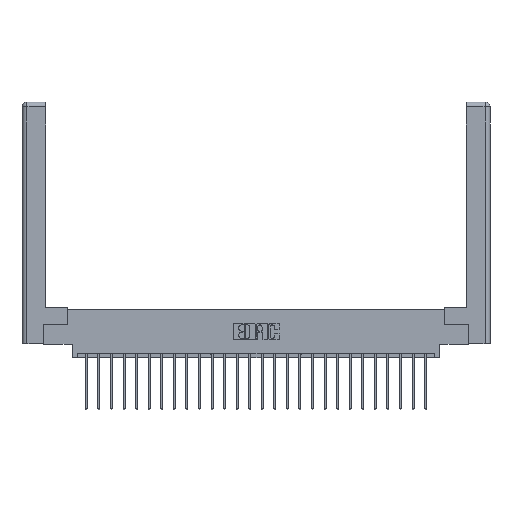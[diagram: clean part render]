
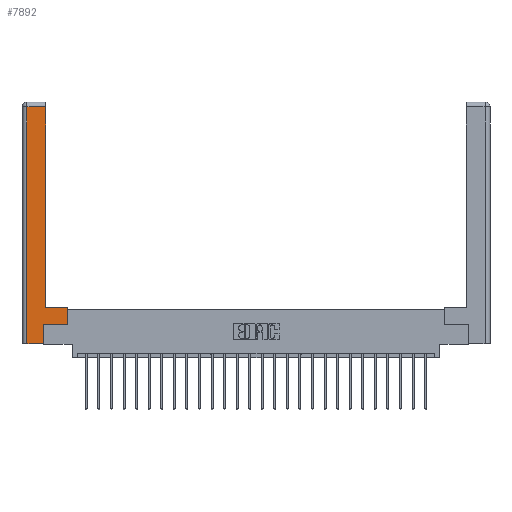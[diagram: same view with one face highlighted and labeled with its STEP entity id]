
A CAD part, top view. The second image highlights one B-rep face of the part: STEP entity #7892.
In plain terms, the highlighted planar face has unit normal (0, 0, 1).
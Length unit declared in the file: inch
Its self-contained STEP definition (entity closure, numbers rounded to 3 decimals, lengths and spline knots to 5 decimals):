
#129 = VECTOR ( 'NONE', #10155, 39.37008 ) ;
#298 = VERTEX_POINT ( 'NONE', #1023 ) ;
#377 = VECTOR ( 'NONE', #16266, 39.37008 ) ;
#504 = CARTESIAN_POINT ( 'NONE',  ( 0.295, 0.45, 0. ) ) ;
#932 = DIRECTION ( 'NONE',  ( 1., 0., 0. ) ) ;
#964 = DIRECTION ( 'NONE',  ( 1., 0., 0. ) ) ;
#1023 = CARTESIAN_POINT ( 'NONE',  ( 0.565, 0.245, 0. ) ) ;
#1202 = VECTOR ( 'NONE', #964, 39.37008 ) ;
#1464 = FACE_OUTER_BOUND ( 'NONE', #13338, .T. ) ;
#1523 = CARTESIAN_POINT ( 'NONE',  ( 0.295, 2.94, 0. ) ) ;
#1764 = VERTEX_POINT ( 'NONE', #23637 ) ;
#1987 = EDGE_CURVE ( 'NONE', #4598, #22615, #16367, .T. ) ;
#2951 = LINE ( 'NONE', #18261, #129 ) ;
#4598 = VERTEX_POINT ( 'NONE', #504 ) ;
#4826 = ORIENTED_EDGE ( 'NONE', *, *, #24903, .T. ) ;
#5138 = EDGE_CURVE ( 'NONE', #13540, #10791, #15281, .T. ) ;
#5182 = LINE ( 'NONE', #15343, #7731 ) ;
#5396 = CARTESIAN_POINT ( 'NONE',  ( 0.0615, 2.94, 0. ) ) ;
#7731 = VECTOR ( 'NONE', #932, 39.37008 ) ;
#7892 = ADVANCED_FACE ( 'NONE', ( #1464 ), #26031, .F. ) ;
#8048 = DIRECTION ( 'NONE',  ( 0., 1., 0. ) ) ;
#8548 = DIRECTION ( 'NONE',  ( 0., 0., -1. ) ) ;
#9258 = LINE ( 'NONE', #14224, #377 ) ;
#9481 = DIRECTION ( 'NONE',  ( -1., 0., 0. ) ) ;
#10155 = DIRECTION ( 'NONE',  ( 0., -1., 0. ) ) ;
#10300 = VECTOR ( 'NONE', #8048, 39.37008 ) ;
#10791 = VERTEX_POINT ( 'NONE', #21172 ) ;
#11776 = VECTOR ( 'NONE', #22174, 39.37008 ) ;
#11961 = VECTOR ( 'NONE', #25441, 39.37008 ) ;
#11969 = VERTEX_POINT ( 'NONE', #19261 ) ;
#12042 = ORIENTED_EDGE ( 'NONE', *, *, #26000, .T. ) ;
#12096 = CARTESIAN_POINT ( 'NONE',  ( 0.295, 3., 0. ) ) ;
#12548 = ORIENTED_EDGE ( 'NONE', *, *, #1987, .T. ) ;
#13338 = EDGE_LOOP ( 'NONE', ( #12548, #18066, #20250, #12042, #24598, #20598, #4826, #26020 ) ) ;
#13540 = VERTEX_POINT ( 'NONE', #19562 ) ;
#13915 = EDGE_CURVE ( 'NONE', #10791, #298, #13944, .T. ) ;
#13944 = LINE ( 'NONE', #25064, #1202 ) ;
#14224 = CARTESIAN_POINT ( 'NONE',  ( 0.295, 0.45, 0. ) ) ;
#14632 = EDGE_CURVE ( 'NONE', #22615, #1764, #26293, .T. ) ;
#14956 = CARTESIAN_POINT ( 'NONE',  ( 0.565, 0.45, 0. ) ) ;
#15281 = LINE ( 'NONE', #22257, #11776 ) ;
#15343 = CARTESIAN_POINT ( 'NONE',  ( 0.265, 0., 0. ) ) ;
#16112 = VECTOR ( 'NONE', #9481, 39.37008 ) ;
#16266 = DIRECTION ( 'NONE',  ( -1., 0., 0. ) ) ;
#16367 = LINE ( 'NONE', #12096, #10300 ) ;
#17189 = CARTESIAN_POINT ( 'NONE',  ( 0.565, 0.45, 0. ) ) ;
#18066 = ORIENTED_EDGE ( 'NONE', *, *, #14632, .T. ) ;
#18261 = CARTESIAN_POINT ( 'NONE',  ( 0.0615, 0., 0. ) ) ;
#18473 = EDGE_CURVE ( 'NONE', #1764, #11969, #2951, .T. ) ;
#19261 = CARTESIAN_POINT ( 'NONE',  ( 0.0615, 0., 0. ) ) ;
#19562 = CARTESIAN_POINT ( 'NONE',  ( 0.265, 0., 0. ) ) ;
#20184 = EDGE_CURVE ( 'NONE', #22266, #4598, #9258, .T. ) ;
#20250 = ORIENTED_EDGE ( 'NONE', *, *, #18473, .T. ) ;
#20385 = CARTESIAN_POINT ( 'NONE',  ( 0., 0., 0. ) ) ;
#20598 = ORIENTED_EDGE ( 'NONE', *, *, #13915, .T. ) ;
#20929 = DIRECTION ( 'NONE',  ( -1., 0., 0. ) ) ;
#21172 = CARTESIAN_POINT ( 'NONE',  ( 0.265, 0.245, 0. ) ) ;
#22174 = DIRECTION ( 'NONE',  ( 0., 1., 0. ) ) ;
#22257 = CARTESIAN_POINT ( 'NONE',  ( 0.265, 0.245, 0. ) ) ;
#22266 = VERTEX_POINT ( 'NONE', #17189 ) ;
#22615 = VERTEX_POINT ( 'NONE', #1523 ) ;
#23637 = CARTESIAN_POINT ( 'NONE',  ( 0.0615, 2.94, 0. ) ) ;
#24057 = LINE ( 'NONE', #14956, #11961 ) ;
#24598 = ORIENTED_EDGE ( 'NONE', *, *, #5138, .T. ) ;
#24680 = AXIS2_PLACEMENT_3D ( 'NONE', #20385, #8548, #20929 ) ;
#24903 = EDGE_CURVE ( 'NONE', #298, #22266, #24057, .T. ) ;
#25064 = CARTESIAN_POINT ( 'NONE',  ( 0.565, 0.245, 0. ) ) ;
#25441 = DIRECTION ( 'NONE',  ( 0., 1., 0. ) ) ;
#26000 = EDGE_CURVE ( 'NONE', #11969, #13540, #5182, .T. ) ;
#26020 = ORIENTED_EDGE ( 'NONE', *, *, #20184, .T. ) ;
#26031 = PLANE ( 'NONE',  #24680 ) ;
#26293 = LINE ( 'NONE', #5396, #16112 ) ;
